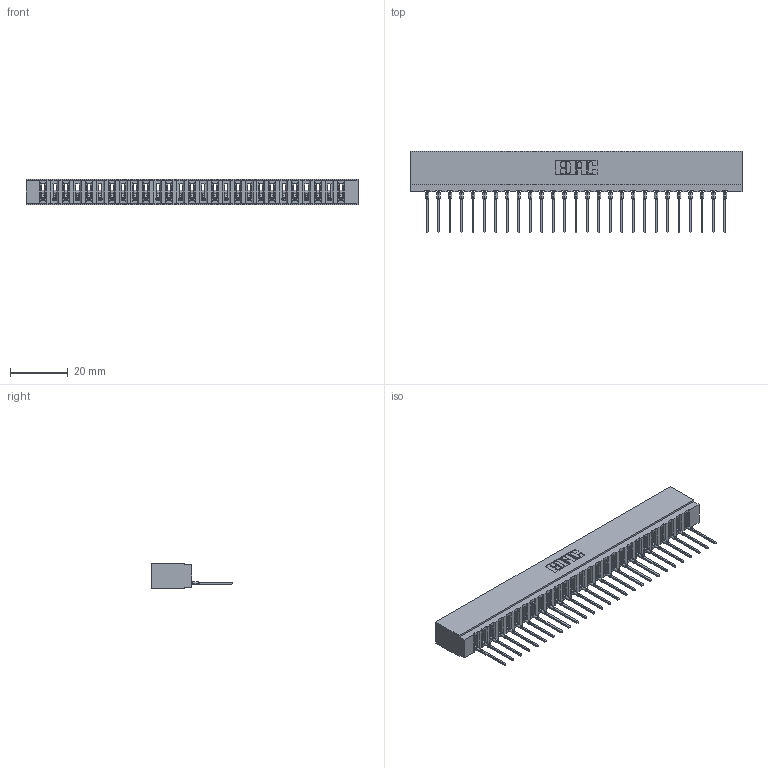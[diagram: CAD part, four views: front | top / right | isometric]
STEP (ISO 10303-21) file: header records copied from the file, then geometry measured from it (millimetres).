
FILE_DESCRIPTION (( 'STEP AP203' ), '1' );
FILE_NAME ('717-027-540-101.STEP', '2026-02-20T21:10:31', ( '' ), ( '' ), 'SwSTEP 2.0', 'SolidWorks 2023', '' );
FILE_SCHEMA (( 'CONFIG_CONTROL_DESIGN' ));
Length unit declared in the file: millimetre
Products named in the file (3): 717-027-540-101; 717 Part_Insulator Option - 06; 745-292-001_540
Assembly tree (28 placements, depth 2):
  717-027-540-101
    717 Part_Insulator Option - 06
    745-292-001_540  x27
Bounding box: 114.86 x 28.18 x 8.89 mm (x, y, z)
Volume: 9829.6 mm3; surface area: 13955.5 mm2
Topology: 28 solids, 28 shells, 3145 faces, 8648 edges, 5458 vertices
Faces by surface type: plane 1890, cylinder 553, bspline 540, torus 162
Entity records: 47461 total; most frequent: CARTESIAN_POINT 8868, ORIENTED_EDGE 8300, DIRECTION 7206, EDGE_CURVE 4150, VECTOR 3806, LINE 3806, VERTEX_POINT 2650, AXIS2_PLACEMENT_3D 1700
